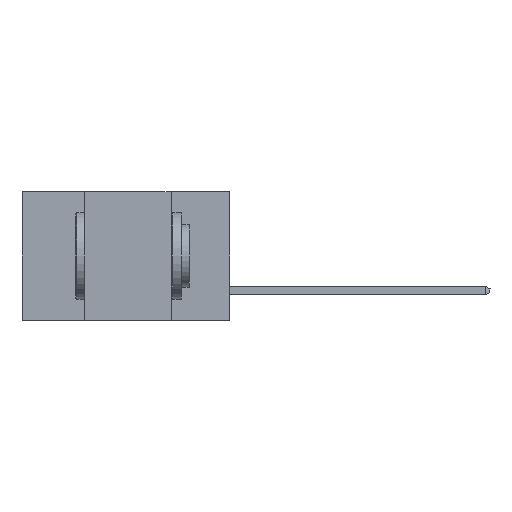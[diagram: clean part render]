
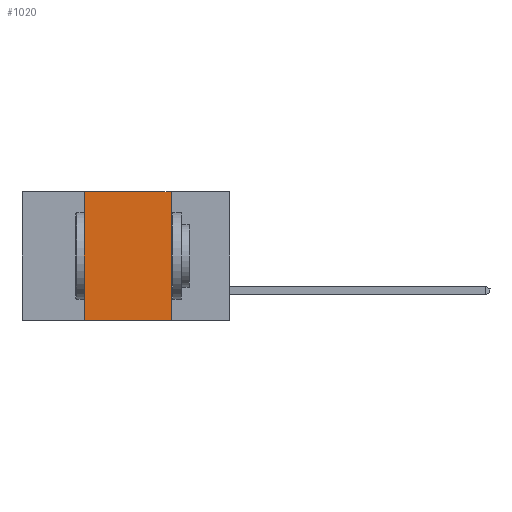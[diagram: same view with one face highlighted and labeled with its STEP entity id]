
A CAD part, left-side view. The second image highlights one B-rep face of the part: STEP entity #1020.
In plain terms, the highlighted planar face has unit normal (-1, 0, 0).
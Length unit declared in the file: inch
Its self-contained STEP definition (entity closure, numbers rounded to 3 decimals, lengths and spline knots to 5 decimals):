
#286 = VERTEX_POINT ( 'NONE', #5285 ) ;
#413 = LINE ( 'NONE', #8687, #4679 ) ;
#471 = VERTEX_POINT ( 'NONE', #8563 ) ;
#557 = DIRECTION ( 'NONE',  ( 0., 0., -1. ) ) ;
#687 = LINE ( 'NONE', #9593, #1533 ) ;
#1020 = ADVANCED_FACE ( 'NONE', ( #1144 ), #9475, .F. ) ;
#1144 = FACE_OUTER_BOUND ( 'NONE', #4638, .T. ) ;
#1199 = AXIS2_PLACEMENT_3D ( 'NONE', #8743, #2028, #8693 ) ;
#1275 = DIRECTION ( 'NONE',  ( 0., -1., 0. ) ) ;
#1533 = VECTOR ( 'NONE', #8715, 39.37008 ) ;
#1723 = CARTESIAN_POINT ( 'NONE',  ( 0., 0.17, 0. ) ) ;
#1885 = DIRECTION ( 'NONE',  ( 0., -1., 0. ) ) ;
#2006 = LINE ( 'NONE', #7942, #6972 ) ;
#2028 = DIRECTION ( 'NONE',  ( 1., 0., 0. ) ) ;
#2183 = EDGE_CURVE ( 'NONE', #471, #286, #687, .T. ) ;
#3123 = EDGE_CURVE ( 'NONE', #5053, #3945, #5840, .T. ) ;
#3315 = ORIENTED_EDGE ( 'NONE', *, *, #9299, .F. ) ;
#3710 = CARTESIAN_POINT ( 'NONE',  ( 0., 0.17, -0.37 ) ) ;
#3945 = VERTEX_POINT ( 'NONE', #3710 ) ;
#4378 = CARTESIAN_POINT ( 'NONE',  ( 0., 0.17, -0.37 ) ) ;
#4638 = EDGE_LOOP ( 'NONE', ( #7841, #3315, #6070, #6516 ) ) ;
#4679 = VECTOR ( 'NONE', #1885, 39.37008 ) ;
#5053 = VERTEX_POINT ( 'NONE', #1723 ) ;
#5285 = CARTESIAN_POINT ( 'NONE',  ( 0., 0.42, 0. ) ) ;
#5840 = LINE ( 'NONE', #4378, #6790 ) ;
#5880 = EDGE_CURVE ( 'NONE', #471, #3945, #413, .T. ) ;
#6070 = ORIENTED_EDGE ( 'NONE', *, *, #2183, .F. ) ;
#6516 = ORIENTED_EDGE ( 'NONE', *, *, #5880, .T. ) ;
#6790 = VECTOR ( 'NONE', #557, 39.37008 ) ;
#6972 = VECTOR ( 'NONE', #1275, 39.37008 ) ;
#7841 = ORIENTED_EDGE ( 'NONE', *, *, #3123, .F. ) ;
#7942 = CARTESIAN_POINT ( 'NONE',  ( 0., 0.6, 0. ) ) ;
#8563 = CARTESIAN_POINT ( 'NONE',  ( 0., 0.42, -0.37 ) ) ;
#8687 = CARTESIAN_POINT ( 'NONE',  ( 0., 0.6, -0.37 ) ) ;
#8693 = DIRECTION ( 'NONE',  ( 0., 0., -1. ) ) ;
#8715 = DIRECTION ( 'NONE',  ( 0., 0., 1. ) ) ;
#8743 = CARTESIAN_POINT ( 'NONE',  ( 0., 0.6, 0. ) ) ;
#9299 = EDGE_CURVE ( 'NONE', #286, #5053, #2006, .T. ) ;
#9475 = PLANE ( 'NONE',  #1199 ) ;
#9593 = CARTESIAN_POINT ( 'NONE',  ( 0., 0.42, -0.37 ) ) ;
